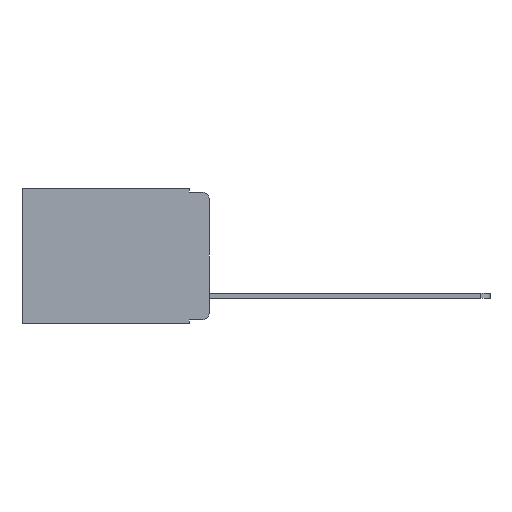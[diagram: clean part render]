
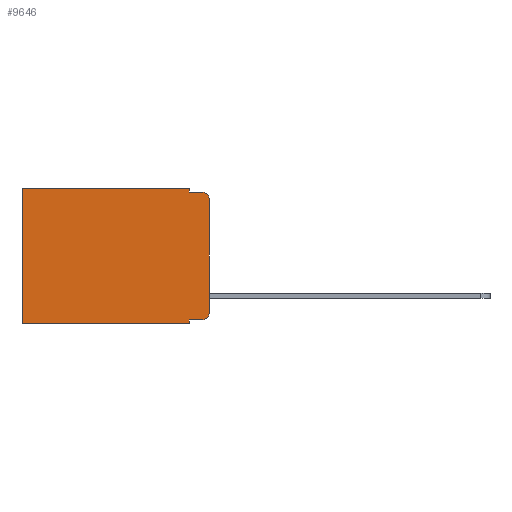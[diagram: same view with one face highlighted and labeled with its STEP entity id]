
A CAD part, left-side view. The second image highlights one B-rep face of the part: STEP entity #9646.
In plain terms, the highlighted planar face has unit normal (-1, 0, 0).
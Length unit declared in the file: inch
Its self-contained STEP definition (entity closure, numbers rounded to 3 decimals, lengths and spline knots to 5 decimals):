
#272 = LINE ( 'NONE', #2949, #8178 ) ;
#279 = CARTESIAN_POINT ( 'NONE',  ( 0.298, 0.02, -0.313 ) ) ;
#284 = VECTOR ( 'NONE', #428, 39.37008 ) ;
#347 = ORIENTED_EDGE ( 'NONE', *, *, #9283, .T. ) ;
#428 = DIRECTION ( 'NONE',  ( 0., -1., 0. ) ) ;
#518 = ORIENTED_EDGE ( 'NONE', *, *, #10408, .F. ) ;
#1191 = VECTOR ( 'NONE', #5348, 39.37008 ) ;
#1248 = PLANE ( 'NONE',  #6690 ) ;
#1268 = AXIS2_PLACEMENT_3D ( 'NONE', #6903, #16733, #8351 ) ;
#1605 = VERTEX_POINT ( 'NONE', #16020 ) ;
#1765 = DIRECTION ( 'NONE',  ( 0., 0., -1. ) ) ;
#1820 = ORIENTED_EDGE ( 'NONE', *, *, #12618, .F. ) ;
#1876 = CARTESIAN_POINT ( 'NONE',  ( 0.298, 0.02, -0.01 ) ) ;
#2079 = ORIENTED_EDGE ( 'NONE', *, *, #3555, .F. ) ;
#2467 = VERTEX_POINT ( 'NONE', #3550 ) ;
#2645 = DIRECTION ( 'NONE',  ( 0., 0., -1. ) ) ;
#2711 = VERTEX_POINT ( 'NONE', #8618 ) ;
#2949 = CARTESIAN_POINT ( 'NONE',  ( 0.298, 0., -0.343 ) ) ;
#3197 = ORIENTED_EDGE ( 'NONE', *, *, #9836, .T. ) ;
#3488 = LINE ( 'NONE', #14067, #18159 ) ;
#3550 = CARTESIAN_POINT ( 'NONE',  ( 0.298, 0.051, -0.343 ) ) ;
#3555 = EDGE_CURVE ( 'NONE', #10231, #18278, #4730, .T. ) ;
#3977 = ORIENTED_EDGE ( 'NONE', *, *, #8297, .F. ) ;
#4269 = CARTESIAN_POINT ( 'NONE',  ( 0.298, 0., 0. ) ) ;
#4472 = CARTESIAN_POINT ( 'NONE',  ( 0.298, 0.051, -0.01 ) ) ;
#4525 = ORIENTED_EDGE ( 'NONE', *, *, #5376, .T. ) ;
#4573 = CARTESIAN_POINT ( 'NONE',  ( 0.298, 0.051, 0. ) ) ;
#4730 = LINE ( 'NONE', #4472, #1191 ) ;
#5348 = DIRECTION ( 'NONE',  ( 0., -1., 0. ) ) ;
#5376 = EDGE_CURVE ( 'NONE', #12750, #11573, #16674, .T. ) ;
#5401 = ORIENTED_EDGE ( 'NONE', *, *, #17290, .T. ) ;
#5817 = VERTEX_POINT ( 'NONE', #14990 ) ;
#5822 = CIRCLE ( 'NONE', #1268, 0.02 ) ;
#6212 = VECTOR ( 'NONE', #14359, 39.37008 ) ;
#6403 = CARTESIAN_POINT ( 'NONE',  ( 0.298, 0.051, -0.333 ) ) ;
#6527 = VERTEX_POINT ( 'NONE', #11962 ) ;
#6690 = AXIS2_PLACEMENT_3D ( 'NONE', #4269, #15696, #7250 ) ;
#6903 = CARTESIAN_POINT ( 'NONE',  ( 0.298, 0.02, -0.03 ) ) ;
#7089 = LINE ( 'NONE', #12454, #13727 ) ;
#7250 = DIRECTION ( 'NONE',  ( 0., 0., -1. ) ) ;
#8178 = VECTOR ( 'NONE', #13080, 39.37008 ) ;
#8297 = EDGE_CURVE ( 'NONE', #13092, #10231, #7089, .T. ) ;
#8351 = DIRECTION ( 'NONE',  ( 0., 0., -1. ) ) ;
#8477 = DIRECTION ( 'NONE',  ( 0., 0., -1. ) ) ;
#8513 = DIRECTION ( 'NONE',  ( 0., 0., -1. ) ) ;
#8618 = CARTESIAN_POINT ( 'NONE',  ( 0.298, 0., -0.03 ) ) ;
#9283 = EDGE_CURVE ( 'NONE', #5817, #1605, #11952, .T. ) ;
#9556 = CIRCLE ( 'NONE', #13314, 0.02 ) ;
#9646 = ADVANCED_FACE ( 'NONE', ( #16318 ), #1248, .F. ) ;
#9752 = VECTOR ( 'NONE', #11885, 39.37008 ) ;
#9807 = CARTESIAN_POINT ( 'NONE',  ( 0.298, 0.473, 0. ) ) ;
#9836 = EDGE_CURVE ( 'NONE', #1605, #6527, #9556, .T. ) ;
#10189 = LINE ( 'NONE', #4573, #9752 ) ;
#10231 = VERTEX_POINT ( 'NONE', #15620 ) ;
#10408 = EDGE_CURVE ( 'NONE', #5817, #2467, #10189, .T. ) ;
#10565 = DIRECTION ( 'NONE',  ( -1., 0., 0. ) ) ;
#11000 = EDGE_CURVE ( 'NONE', #2467, #11573, #272, .T. ) ;
#11573 = VERTEX_POINT ( 'NONE', #18572 ) ;
#11654 = ORIENTED_EDGE ( 'NONE', *, *, #15440, .T. ) ;
#11865 = CARTESIAN_POINT ( 'NONE',  ( 0.298, 0.473, 0. ) ) ;
#11885 = DIRECTION ( 'NONE',  ( 0., 0., -1. ) ) ;
#11952 = LINE ( 'NONE', #6403, #284 ) ;
#11962 = CARTESIAN_POINT ( 'NONE',  ( 0.298, 0., -0.313 ) ) ;
#12454 = CARTESIAN_POINT ( 'NONE',  ( 0.298, 0.051, 0. ) ) ;
#12618 = EDGE_CURVE ( 'NONE', #2711, #6527, #3488, .T. ) ;
#12750 = VERTEX_POINT ( 'NONE', #11865 ) ;
#12950 = CARTESIAN_POINT ( 'NONE',  ( 0.298, 0., 0. ) ) ;
#13080 = DIRECTION ( 'NONE',  ( 0., 1., 0. ) ) ;
#13092 = VERTEX_POINT ( 'NONE', #15399 ) ;
#13150 = ORIENTED_EDGE ( 'NONE', *, *, #11000, .F. ) ;
#13314 = AXIS2_PLACEMENT_3D ( 'NONE', #279, #10565, #1765 ) ;
#13727 = VECTOR ( 'NONE', #8513, 39.37008 ) ;
#13741 = LINE ( 'NONE', #12950, #6212 ) ;
#14067 = CARTESIAN_POINT ( 'NONE',  ( 0.298, 0., 0. ) ) ;
#14359 = DIRECTION ( 'NONE',  ( 0., 1., 0. ) ) ;
#14990 = CARTESIAN_POINT ( 'NONE',  ( 0.298, 0.051, -0.333 ) ) ;
#15385 = VECTOR ( 'NONE', #2645, 39.37008 ) ;
#15399 = CARTESIAN_POINT ( 'NONE',  ( 0.298, 0.051, 0. ) ) ;
#15440 = EDGE_CURVE ( 'NONE', #13092, #12750, #13741, .T. ) ;
#15620 = CARTESIAN_POINT ( 'NONE',  ( 0.298, 0.051, -0.01 ) ) ;
#15696 = DIRECTION ( 'NONE',  ( 1., 0., 0. ) ) ;
#16020 = CARTESIAN_POINT ( 'NONE',  ( 0.298, 0.02, -0.333 ) ) ;
#16026 = EDGE_LOOP ( 'NONE', ( #1820, #5401, #2079, #3977, #11654, #4525, #13150, #518, #347, #3197 ) ) ;
#16318 = FACE_OUTER_BOUND ( 'NONE', #16026, .T. ) ;
#16674 = LINE ( 'NONE', #9807, #15385 ) ;
#16733 = DIRECTION ( 'NONE',  ( -1., 0., 0. ) ) ;
#17290 = EDGE_CURVE ( 'NONE', #2711, #18278, #5822, .T. ) ;
#18159 = VECTOR ( 'NONE', #8477, 39.37008 ) ;
#18278 = VERTEX_POINT ( 'NONE', #1876 ) ;
#18572 = CARTESIAN_POINT ( 'NONE',  ( 0.298, 0.473, -0.343 ) ) ;
